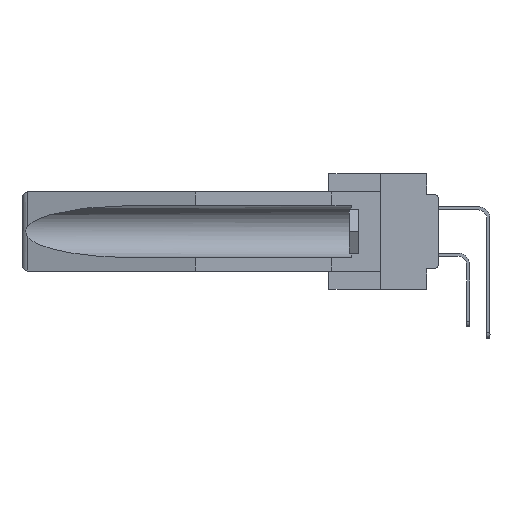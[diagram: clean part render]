
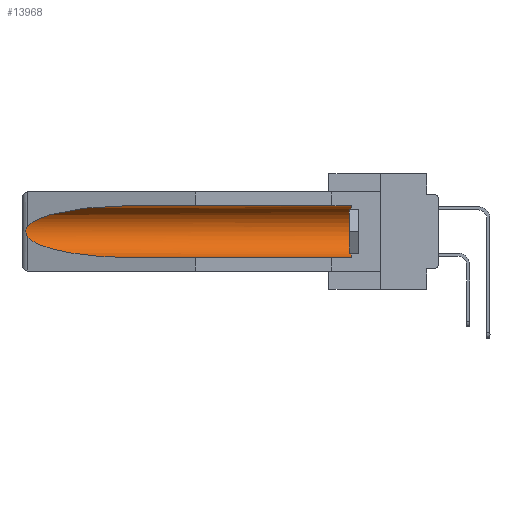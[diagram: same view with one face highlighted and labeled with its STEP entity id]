
A CAD part, left-side view. The second image highlights one B-rep face of the part: STEP entity #13968.
In plain terms, the highlighted cylindrical face has radius 2.857 mm (diameter 5.715 mm), a partial arc.
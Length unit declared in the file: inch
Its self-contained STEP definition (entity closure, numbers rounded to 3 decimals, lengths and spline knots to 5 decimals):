
#82 = CARTESIAN_POINT ( 'NONE',  ( 0.155, 1.07973, -0.284 ) ) ;
#135 = VERTEX_POINT ( 'NONE', #19210 ) ;
#859 = DIRECTION ( 'NONE',  ( 0., 1., 0. ) ) ;
#918 = ORIENTED_EDGE ( 'NONE', *, *, #7662, .T. ) ;
#1068 = DIRECTION ( 'NONE',  ( 0., 1., 0. ) ) ;
#1222 =( BOUNDED_CURVE ( )  B_SPLINE_CURVE ( 3, ( #24232, #32257, #2699, #5018 ),
 .UNSPECIFIED., .F., .F. ) 
 B_SPLINE_CURVE_WITH_KNOTS ( ( 4, 4 ),
 ( 4.71239, 6.08839 ),
 .UNSPECIFIED. ) 
 CURVE ( )  GEOMETRIC_REPRESENTATION_ITEM ( )  RATIONAL_B_SPLINE_CURVE ( ( 1., 0.848, 0.848, 1. ) ) 
 REPRESENTATION_ITEM ( '' )  );
#1284 = CARTESIAN_POINT ( 'NONE',  ( 0.26537, 1.52718, -0.14972 ) ) ;
#2699 = CARTESIAN_POINT ( 'NONE',  ( 0.25451, 1.48313, -0.09465 ) ) ;
#3329 = VERTEX_POINT ( 'NONE', #14717 ) ;
#3965 = CARTESIAN_POINT ( 'NONE',  ( 0.26537, 1.52718, -0.19328 ) ) ;
#5018 = CARTESIAN_POINT ( 'NONE',  ( 0.26537, 1.52718, -0.14972 ) ) ;
#5301 = AXIS2_PLACEMENT_3D ( 'NONE', #28296, #1068, #9427 ) ;
#5760 = VECTOR ( 'NONE', #859, 39.37008 ) ;
#6293 = VERTEX_POINT ( 'NONE', #9512 ) ;
#6619 = CARTESIAN_POINT ( 'NONE',  ( 0.2673, 1.5327, -0.16383 ) ) ;
#6631 = EDGE_CURVE ( 'NONE', #135, #12028, #26661, .T. ) ;
#7662 = EDGE_CURVE ( 'NONE', #12028, #29028, #32833, .T. ) ;
#8128 = EDGE_CURVE ( 'NONE', #19522, #135, #1222, .T. ) ;
#8169 = CIRCLE ( 'NONE', #28061, 0.1125 ) ;
#8424 = CARTESIAN_POINT ( 'NONE',  ( 0.26537, 1.52718, -0.19328 ) ) ;
#9250 = CYLINDRICAL_SURFACE ( 'NONE', #5301, 0.1125 ) ;
#9300 = CARTESIAN_POINT ( 'NONE',  ( 0.2675, 1.53308, -0.17534 ) ) ;
#9427 = DIRECTION ( 'NONE',  ( 0., 0., 1. ) ) ;
#9512 = CARTESIAN_POINT ( 'NONE',  ( 0.155, 0.126, -0.284 ) ) ;
#9558 = EDGE_CURVE ( 'NONE', #6293, #29028, #34735, .T. ) ;
#9671 = ORIENTED_EDGE ( 'NONE', *, *, #16385, .T. ) ;
#10719 = CARTESIAN_POINT ( 'NONE',  ( 0.155, -0.30754, -0.284 ) ) ;
#12028 = VERTEX_POINT ( 'NONE', #25978 ) ;
#12465 = EDGE_CURVE ( 'NONE', #3329, #19522, #25409, .T. ) ;
#13074 = CARTESIAN_POINT ( 'NONE',  ( 0.155, 0.126, -0.1715 ) ) ;
#13666 = VECTOR ( 'NONE', #21578, 39.37008 ) ;
#13968 = ADVANCED_FACE ( 'NONE', ( #28122 ), #9250, .F. ) ;
#14717 = CARTESIAN_POINT ( 'NONE',  ( 0.155, 0.126, -0.059 ) ) ;
#14990 = CARTESIAN_POINT ( 'NONE',  ( 0.26654, 1.53092, -0.15636 ) ) ;
#16385 = EDGE_CURVE ( 'NONE', #6293, #3329, #8169, .T. ) ;
#16487 = CARTESIAN_POINT ( 'NONE',  ( 0.155, 1.07973, -0.284 ) ) ;
#16855 = CARTESIAN_POINT ( 'NONE',  ( 0.155, 1.07973, -0.059 ) ) ;
#17238 = EDGE_LOOP ( 'NONE', ( #19607, #17318, #918, #34928, #9671, #18580 ) ) ;
#17318 = ORIENTED_EDGE ( 'NONE', *, *, #6631, .T. ) ;
#18580 = ORIENTED_EDGE ( 'NONE', *, *, #12465, .T. ) ;
#19210 = CARTESIAN_POINT ( 'NONE',  ( 0.26537, 1.52718, -0.14972 ) ) ;
#19522 = VERTEX_POINT ( 'NONE', #16855 ) ;
#19607 = ORIENTED_EDGE ( 'NONE', *, *, #8128, .T. ) ;
#20512 = CARTESIAN_POINT ( 'NONE',  ( 0.26597, 1.52961, -0.15275 ) ) ;
#21578 = DIRECTION ( 'NONE',  ( 0., 1., 0. ) ) ;
#23925 = DIRECTION ( 'NONE',  ( 0., -1., 0. ) ) ;
#24232 = CARTESIAN_POINT ( 'NONE',  ( 0.155, 1.07973, -0.059 ) ) ;
#25409 = LINE ( 'NONE', #25588, #5760 ) ;
#25588 = CARTESIAN_POINT ( 'NONE',  ( 0.155, -0.30754, -0.059 ) ) ;
#25665 = CARTESIAN_POINT ( 'NONE',  ( 0.2675, 1.53308, -0.16763 ) ) ;
#25978 = CARTESIAN_POINT ( 'NONE',  ( 0.26537, 1.52718, -0.19328 ) ) ;
#26661 = B_SPLINE_CURVE_WITH_KNOTS ( 'NONE', 3,
 ( #1284, #20512, #14990, #6619, #25665, #9300, #31186, #28696, #28348, #3965 ),
 .UNSPECIFIED., .F., .F.,
 ( 4, 2, 2, 2, 4 ),
 ( 0., 0.00029, 0.00058, 0.00087, 0.00117 ),
 .UNSPECIFIED. ) ;
#26949 = CARTESIAN_POINT ( 'NONE',  ( 0.25451, 1.48313, -0.24835 ) ) ;
#28061 = AXIS2_PLACEMENT_3D ( 'NONE', #13074, #23925, #34088 ) ;
#28122 = FACE_OUTER_BOUND ( 'NONE', #17238, .T. ) ;
#28296 = CARTESIAN_POINT ( 'NONE',  ( 0.155, -0.30754, -0.1715 ) ) ;
#28348 = CARTESIAN_POINT ( 'NONE',  ( 0.26597, 1.5296, -0.19026 ) ) ;
#28696 = CARTESIAN_POINT ( 'NONE',  ( 0.26655, 1.53094, -0.18657 ) ) ;
#29028 = VERTEX_POINT ( 'NONE', #16487 ) ;
#29447 = CARTESIAN_POINT ( 'NONE',  ( 0.21114, 1.30732, -0.284 ) ) ;
#31186 = CARTESIAN_POINT ( 'NONE',  ( 0.2673, 1.53269, -0.17917 ) ) ;
#32257 = CARTESIAN_POINT ( 'NONE',  ( 0.21114, 1.30732, -0.059 ) ) ;
#32833 =( BOUNDED_CURVE ( )  B_SPLINE_CURVE ( 3, ( #8424, #26949, #29447, #82 ),
 .UNSPECIFIED., .F., .T. ) 
 B_SPLINE_CURVE_WITH_KNOTS ( ( 4, 4 ),
 ( 0.1948, 1.5708 ),
 .UNSPECIFIED. ) 
 CURVE ( )  GEOMETRIC_REPRESENTATION_ITEM ( )  RATIONAL_B_SPLINE_CURVE ( ( 1., 0.848, 0.848, 1. ) ) 
 REPRESENTATION_ITEM ( '' )  );
#34088 = DIRECTION ( 'NONE',  ( 0., 0., 1. ) ) ;
#34735 = LINE ( 'NONE', #10719, #13666 ) ;
#34928 = ORIENTED_EDGE ( 'NONE', *, *, #9558, .F. ) ;
